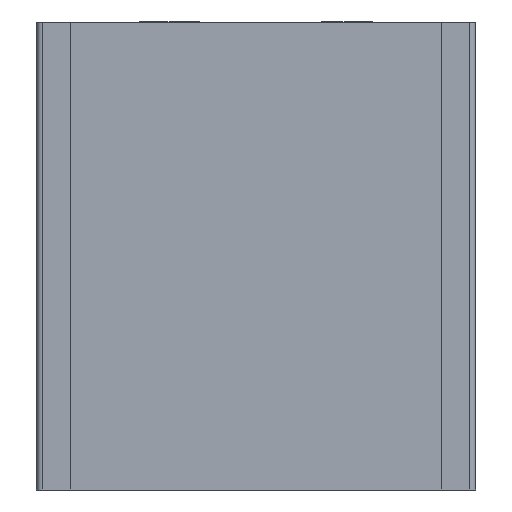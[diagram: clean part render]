
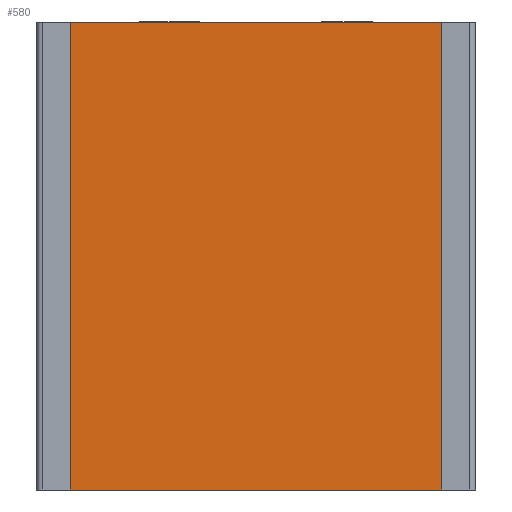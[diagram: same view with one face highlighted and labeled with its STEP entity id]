
A CAD part, front view. The second image highlights one B-rep face of the part: STEP entity #580.
In plain terms, the highlighted planar face has unit normal (0, -1, 0).
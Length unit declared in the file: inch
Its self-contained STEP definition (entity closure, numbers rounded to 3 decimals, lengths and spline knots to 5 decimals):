
#32=PLANE('',#636);
#50=FACE_OUTER_BOUND('',#80,.T.);
#80=EDGE_LOOP('',(#402,#403,#404,#405));
#118=LINE('',#867,#173);
#119=LINE('',#869,#174);
#120=LINE('',#871,#175);
#121=LINE('',#872,#176);
#173=VECTOR('',#704,0.3937);
#174=VECTOR('',#705,0.3937);
#175=VECTOR('',#706,0.3937);
#176=VECTOR('',#707,0.3937);
#254=VERTEX_POINT('',#865);
#255=VERTEX_POINT('',#866);
#256=VERTEX_POINT('',#868);
#257=VERTEX_POINT('',#870);
#314=EDGE_CURVE('',#254,#255,#118,.T.);
#315=EDGE_CURVE('',#256,#254,#119,.T.);
#316=EDGE_CURVE('',#257,#256,#120,.T.);
#317=EDGE_CURVE('',#255,#257,#121,.T.);
#402=ORIENTED_EDGE('',*,*,#314,.F.);
#403=ORIENTED_EDGE('',*,*,#315,.F.);
#404=ORIENTED_EDGE('',*,*,#316,.F.);
#405=ORIENTED_EDGE('',*,*,#317,.F.);
#580=ADVANCED_FACE('',(#50),#32,.F.);
#636=AXIS2_PLACEMENT_3D('',#864,#702,#703);
#702=DIRECTION('center_axis',(0.,1.,0.));
#703=DIRECTION('ref_axis',(0.,0.,1.));
#704=DIRECTION('',(-1.,0.,0.));
#705=DIRECTION('',(0.,0.,-1.));
#706=DIRECTION('',(1.,0.,0.));
#707=DIRECTION('',(0.,0.,1.));
#864=CARTESIAN_POINT('Origin',(-0.314,-0.44022,-0.74852));
#865=CARTESIAN_POINT('',(0.314,-0.44022,-0.431));
#866=CARTESIAN_POINT('',(-0.314,-0.44022,-0.431));
#867=CARTESIAN_POINT('',(0.09761,-0.44022,-0.431));
#868=CARTESIAN_POINT('',(0.314,-0.44022,0.361));
#869=CARTESIAN_POINT('',(0.314,-0.44022,-2.46337));
#870=CARTESIAN_POINT('',(-0.314,-0.44022,0.361));
#871=CARTESIAN_POINT('',(0.0335,-0.44022,0.361));
#872=CARTESIAN_POINT('',(-0.314,-0.44022,-2.46337));
